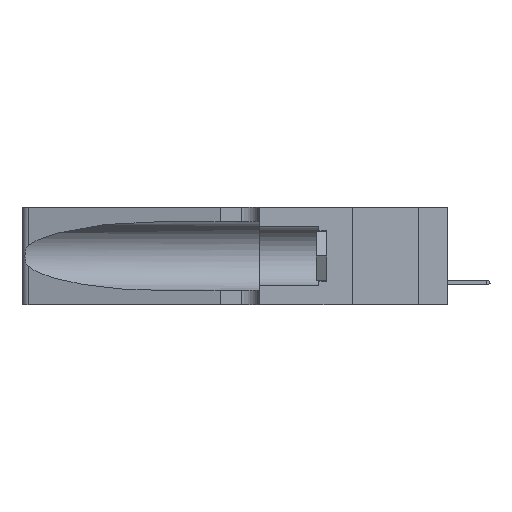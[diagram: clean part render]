
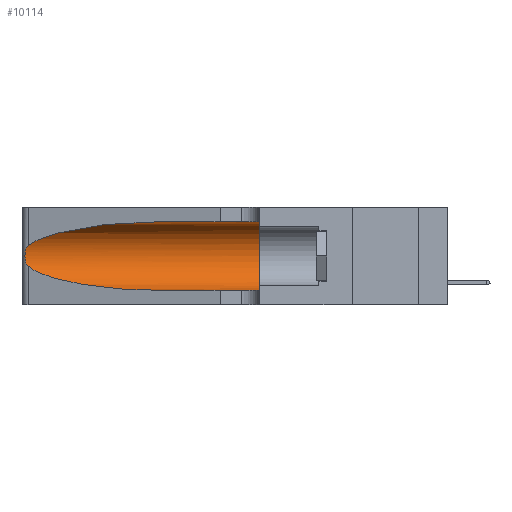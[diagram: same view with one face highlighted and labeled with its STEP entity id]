
A CAD part, left-side view. The second image highlights one B-rep face of the part: STEP entity #10114.
In plain terms, the highlighted cylindrical face has radius 3.308 mm (diameter 6.617 mm), a partial arc.
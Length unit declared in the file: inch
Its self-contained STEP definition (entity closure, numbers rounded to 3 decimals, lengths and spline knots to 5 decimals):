
#871 = AXIS2_PLACEMENT_3D ( 'NONE', #34248, #15465, #34567 ) ;
#1142 = CARTESIAN_POINT ( 'NONE',  ( 0.25487, 1.22718, 0.22369 ) ) ;
#3492 = CARTESIAN_POINT ( 'NONE',  ( 0.25787, 1.23484, 0.2124 ) ) ;
#4921 = CARTESIAN_POINT ( 'NONE',  ( 0.25487, 1.22718, 0.14631 ) ) ;
#4981 = ORIENTED_EDGE ( 'NONE', *, *, #30117, .F. ) ;
#5011 = CARTESIAN_POINT ( 'NONE',  ( 0.26018, 1.23835, 0.19895 ) ) ;
#5076 = CARTESIAN_POINT ( 'NONE',  ( 0.2373, 1.15595, 0.28018 ) ) ;
#6738 = CARTESIAN_POINT ( 'NONE',  ( 0.25639, 1.23186, 0.15144 ) ) ;
#7213 =( BOUNDED_CURVE ( )  B_SPLINE_CURVE ( 3, ( #4921, #35220, #12474, #20000 ),
 .UNSPECIFIED., .F., .T. ) 
 B_SPLINE_CURVE_WITH_KNOTS ( ( 4, 4 ),
 ( 3.44316, 4.71239 ),
 .UNSPECIFIED. ) 
 CURVE ( )  GEOMETRIC_REPRESENTATION_ITEM ( )  RATIONAL_B_SPLINE_CURVE ( ( 1., 0.87, 0.87, 1. ) ) 
 REPRESENTATION_ITEM ( '' )  );
#7537 = CARTESIAN_POINT ( 'NONE',  ( 0.25555, 1.22993, 0.14849 ) ) ;
#8151 = ORIENTED_EDGE ( 'NONE', *, *, #42721, .T. ) ;
#8220 = CARTESIAN_POINT ( 'NONE',  ( 0.18966, 0.96281, 0.31525 ) ) ;
#10114 = ADVANCED_FACE ( 'NONE', ( #29810 ), #35107, .F. ) ;
#10370 = EDGE_CURVE ( 'NONE', #42681, #45496, #7213, .T. ) ;
#10746 = CARTESIAN_POINT ( 'NONE',  ( 0.26075, 1.23896, 0.19203 ) ) ;
#11615 = CARTESIAN_POINT ( 'NONE',  ( 0.25487, 1.22718, 0.14631 ) ) ;
#12474 = CARTESIAN_POINT ( 'NONE',  ( 0.18966, 0.96281, 0.05475 ) ) ;
#13599 = DIRECTION ( 'NONE',  ( 0., -1., 0. ) ) ;
#15465 = DIRECTION ( 'NONE',  ( 0., 1., 0. ) ) ;
#15970 = ORIENTED_EDGE ( 'NONE', *, *, #33620, .T. ) ;
#16452 = VERTEX_POINT ( 'NONE', #20585 ) ;
#16659 = VECTOR ( 'NONE', #42816, 39.37008 ) ;
#16727 = ORIENTED_EDGE ( 'NONE', *, *, #10370, .T. ) ;
#17412 = EDGE_CURVE ( 'NONE', #45496, #48697, #20039, .T. ) ;
#17918 = CARTESIAN_POINT ( 'NONE',  ( 0.1305, 1.61858, 0.185 ) ) ;
#17982 = CARTESIAN_POINT ( 'NONE',  ( 0.25487, 1.22718, 0.22369 ) ) ;
#18264 = CARTESIAN_POINT ( 'NONE',  ( 0.1305, 0.72297, 0.05475 ) ) ;
#18739 = CARTESIAN_POINT ( 'NONE',  ( 0.1305, 1.61858, 0.31525 ) ) ;
#20000 = CARTESIAN_POINT ( 'NONE',  ( 0.1305, 0.72297, 0.05475 ) ) ;
#20039 = LINE ( 'NONE', #25002, #41919 ) ;
#20482 = CARTESIAN_POINT ( 'NONE',  ( 0.1305, 0.35, 0.05475 ) ) ;
#20585 = CARTESIAN_POINT ( 'NONE',  ( 0.25487, 1.22718, 0.22369 ) ) ;
#25002 = CARTESIAN_POINT ( 'NONE',  ( 0.1305, 1.61858, 0.05475 ) ) ;
#25621 = CARTESIAN_POINT ( 'NONE',  ( 0.1305, 0.72297, 0.31525 ) ) ;
#26171 = ORIENTED_EDGE ( 'NONE', *, *, #17412, .T. ) ;
#29139 = CARTESIAN_POINT ( 'NONE',  ( 0.26075, 1.23896, 0.178 ) ) ;
#29523 = CARTESIAN_POINT ( 'NONE',  ( 0.25487, 1.22718, 0.14631 ) ) ;
#29810 = FACE_OUTER_BOUND ( 'NONE', #46960, .T. ) ;
#30117 = EDGE_CURVE ( 'NONE', #32349, #48697, #44898, .T. ) ;
#30141 = CARTESIAN_POINT ( 'NONE',  ( 0.1305, 0.35, 0.31525 ) ) ;
#30405 = B_SPLINE_CURVE_WITH_KNOTS ( 'NONE', 3,
 ( #17982, #40323, #46136, #3492, #30834, #5011, #10746, #29139, #48134, #44499, #31219, #6738, #7537, #11615 ),
 .UNSPECIFIED., .F., .F.,
 ( 4, 2, 2, 2, 2, 2, 4 ),
 ( 0., 0.00027, 0.00053, 0.00107, 0.0016, 0.00187, 0.00214 ),
 .UNSPECIFIED. ) ;
#30834 = CARTESIAN_POINT ( 'NONE',  ( 0.25854, 1.2359, 0.20912 ) ) ;
#31219 = CARTESIAN_POINT ( 'NONE',  ( 0.25789, 1.23486, 0.15765 ) ) ;
#32349 = VERTEX_POINT ( 'NONE', #30141 ) ;
#33531 = ORIENTED_EDGE ( 'NONE', *, *, #45992, .F. ) ;
#33620 = EDGE_CURVE ( 'NONE', #37340, #16452, #48622, .T. ) ;
#34248 = CARTESIAN_POINT ( 'NONE',  ( 0.1305, 0.35, 0.185 ) ) ;
#34567 = DIRECTION ( 'NONE',  ( 0., 0., 1. ) ) ;
#35107 = CYLINDRICAL_SURFACE ( 'NONE', #38195, 0.13025 ) ;
#35220 = CARTESIAN_POINT ( 'NONE',  ( 0.2373, 1.15595, 0.08982 ) ) ;
#37340 = VERTEX_POINT ( 'NONE', #25621 ) ;
#38195 = AXIS2_PLACEMENT_3D ( 'NONE', #17918, #41202, #44505 ) ;
#40323 = CARTESIAN_POINT ( 'NONE',  ( 0.25555, 1.22994, 0.2215 ) ) ;
#41202 = DIRECTION ( 'NONE',  ( 0., -1., 0. ) ) ;
#41919 = VECTOR ( 'NONE', #13599, 39.37008 ) ;
#42681 = VERTEX_POINT ( 'NONE', #29523 ) ;
#42721 = EDGE_CURVE ( 'NONE', #16452, #42681, #30405, .T. ) ;
#42816 = DIRECTION ( 'NONE',  ( 0., -1., 0. ) ) ;
#44499 = CARTESIAN_POINT ( 'NONE',  ( 0.25856, 1.23593, 0.16098 ) ) ;
#44505 = DIRECTION ( 'NONE',  ( 0., 0., -1. ) ) ;
#44898 = CIRCLE ( 'NONE', #871, 0.13025 ) ;
#45496 = VERTEX_POINT ( 'NONE', #18264 ) ;
#45992 = EDGE_CURVE ( 'NONE', #37340, #32349, #48010, .T. ) ;
#46136 = CARTESIAN_POINT ( 'NONE',  ( 0.25639, 1.23184, 0.21858 ) ) ;
#46247 = CARTESIAN_POINT ( 'NONE',  ( 0.1305, 0.72297, 0.31525 ) ) ;
#46960 = EDGE_LOOP ( 'NONE', ( #15970, #8151, #16727, #26171, #4981, #33531 ) ) ;
#48010 = LINE ( 'NONE', #18739, #16659 ) ;
#48134 = CARTESIAN_POINT ( 'NONE',  ( 0.26017, 1.23833, 0.17102 ) ) ;
#48622 =( BOUNDED_CURVE ( )  B_SPLINE_CURVE ( 3, ( #46247, #8220, #5076, #1142 ),
 .UNSPECIFIED., .F., .F. ) 
 B_SPLINE_CURVE_WITH_KNOTS ( ( 4, 4 ),
 ( 1.5708, 2.84003 ),
 .UNSPECIFIED. ) 
 CURVE ( )  GEOMETRIC_REPRESENTATION_ITEM ( )  RATIONAL_B_SPLINE_CURVE ( ( 1., 0.87, 0.87, 1. ) ) 
 REPRESENTATION_ITEM ( '' )  );
#48697 = VERTEX_POINT ( 'NONE', #20482 ) ;
